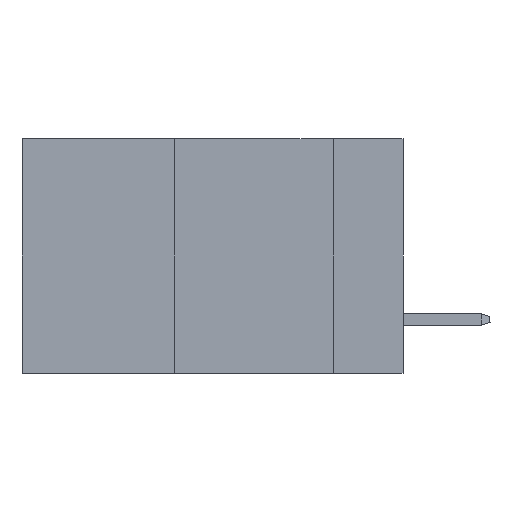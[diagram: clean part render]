
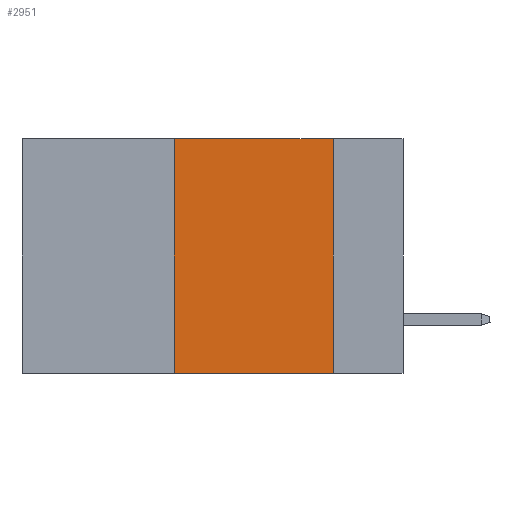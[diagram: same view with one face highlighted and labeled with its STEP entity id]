
A CAD part, left-side view. The second image highlights one B-rep face of the part: STEP entity #2951.
In plain terms, the highlighted planar face has unit normal (-1, 0, 0).
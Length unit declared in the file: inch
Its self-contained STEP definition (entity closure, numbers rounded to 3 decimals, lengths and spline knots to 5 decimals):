
#516 = EDGE_CURVE ( 'NONE', #1204, #9489, #17212, .T. ) ;
#710 = LINE ( 'NONE', #10046, #5634 ) ;
#1204 = VERTEX_POINT ( 'NONE', #16892 ) ;
#2951 = ADVANCED_FACE ( 'NONE', ( #11767 ), #19423, .F. ) ;
#3224 = LINE ( 'NONE', #10614, #13418 ) ;
#3418 = AXIS2_PLACEMENT_3D ( 'NONE', #3963, #14411, #10042 ) ;
#3447 = VERTEX_POINT ( 'NONE', #13469 ) ;
#3963 = CARTESIAN_POINT ( 'NONE',  ( 0., 0.6, 0. ) ) ;
#4280 = EDGE_CURVE ( 'NONE', #9078, #1204, #710, .T. ) ;
#4612 = ORIENTED_EDGE ( 'NONE', *, *, #12029, .T. ) ;
#4860 = ORIENTED_EDGE ( 'NONE', *, *, #14075, .F. ) ;
#5214 = CARTESIAN_POINT ( 'NONE',  ( 0., 0.6, 0. ) ) ;
#5634 = VECTOR ( 'NONE', #6919, 39.37008 ) ;
#6162 = CARTESIAN_POINT ( 'NONE',  ( 0., 0.11, 0. ) ) ;
#6919 = DIRECTION ( 'NONE',  ( 0., 0., 1. ) ) ;
#7878 = DIRECTION ( 'NONE',  ( 0., -1., 0. ) ) ;
#7976 = DIRECTION ( 'NONE',  ( 0., -1., 0. ) ) ;
#8719 = CARTESIAN_POINT ( 'NONE',  ( 0., 0.36, -0.37 ) ) ;
#9077 = EDGE_LOOP ( 'NONE', ( #4860, #10465, #12662, #4612 ) ) ;
#9078 = VERTEX_POINT ( 'NONE', #8719 ) ;
#9489 = VERTEX_POINT ( 'NONE', #6162 ) ;
#10042 = DIRECTION ( 'NONE',  ( 0., 0., -1. ) ) ;
#10046 = CARTESIAN_POINT ( 'NONE',  ( 0., 0.36, 0. ) ) ;
#10465 = ORIENTED_EDGE ( 'NONE', *, *, #516, .F. ) ;
#10614 = CARTESIAN_POINT ( 'NONE',  ( 0., 0.6, -0.37 ) ) ;
#11429 = VECTOR ( 'NONE', #7976, 39.37008 ) ;
#11767 = FACE_OUTER_BOUND ( 'NONE', #9077, .T. ) ;
#12029 = EDGE_CURVE ( 'NONE', #9078, #3447, #3224, .T. ) ;
#12662 = ORIENTED_EDGE ( 'NONE', *, *, #4280, .F. ) ;
#13418 = VECTOR ( 'NONE', #7878, 39.37008 ) ;
#13469 = CARTESIAN_POINT ( 'NONE',  ( 0., 0.11, -0.37 ) ) ;
#14075 = EDGE_CURVE ( 'NONE', #9489, #3447, #18683, .T. ) ;
#14411 = DIRECTION ( 'NONE',  ( 1., 0., 0. ) ) ;
#16892 = CARTESIAN_POINT ( 'NONE',  ( 0., 0.36, 0. ) ) ;
#17212 = LINE ( 'NONE', #5214, #11429 ) ;
#17250 = DIRECTION ( 'NONE',  ( 0., 0., -1. ) ) ;
#18683 = LINE ( 'NONE', #18880, #18977 ) ;
#18880 = CARTESIAN_POINT ( 'NONE',  ( 0., 0.11, 0. ) ) ;
#18977 = VECTOR ( 'NONE', #17250, 39.37008 ) ;
#19423 = PLANE ( 'NONE',  #3418 ) ;
